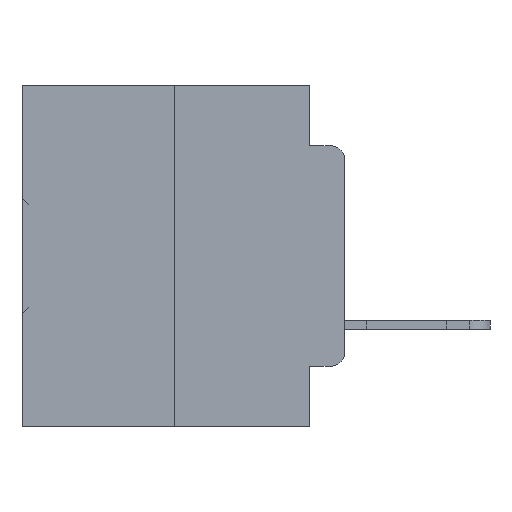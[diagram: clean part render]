
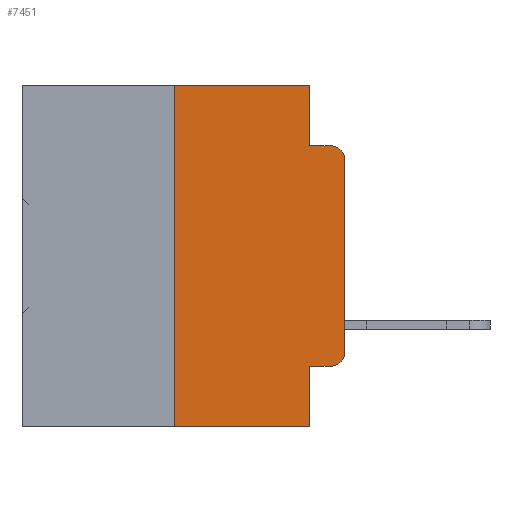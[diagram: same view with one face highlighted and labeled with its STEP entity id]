
A CAD part, left-side view. The second image highlights one B-rep face of the part: STEP entity #7451.
In plain terms, the highlighted planar face has unit normal (-1, 0, 0).
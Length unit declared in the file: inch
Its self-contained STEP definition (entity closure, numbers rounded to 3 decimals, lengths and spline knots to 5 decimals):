
#826 = EDGE_LOOP ( 'NONE', ( #3162, #15771, #3826, #35376, #5031, #7640, #29215, #8530, #10834, #23584 ) ) ;
#985 = VERTEX_POINT ( 'NONE', #22068 ) ;
#1111 = VECTOR ( 'NONE', #28301, 39.37008 ) ;
#1576 = DIRECTION ( 'NONE',  ( 0., 0., -1. ) ) ;
#1656 = DIRECTION ( 'NONE',  ( 0., 0., -1. ) ) ;
#1663 = DIRECTION ( 'NONE',  ( 1., 0., 0. ) ) ;
#1795 = PLANE ( 'NONE',  #16430 ) ;
#1800 = EDGE_CURVE ( 'NONE', #10800, #985, #11108, .T. ) ;
#1982 = VECTOR ( 'NONE', #33667, 39.37008 ) ;
#2269 = CARTESIAN_POINT ( 'NONE',  ( 0., 0.473, 0. ) ) ;
#2577 = VERTEX_POINT ( 'NONE', #4134 ) ;
#2790 = VECTOR ( 'NONE', #16209, 39.37008 ) ;
#3162 = ORIENTED_EDGE ( 'NONE', *, *, #30580, .T. ) ;
#3176 = VECTOR ( 'NONE', #31757, 39.37008 ) ;
#3826 = ORIENTED_EDGE ( 'NONE', *, *, #15657, .F. ) ;
#4134 = CARTESIAN_POINT ( 'NONE',  ( 0., 0.02, -0.4115 ) ) ;
#4499 = LINE ( 'NONE', #11227, #1982 ) ;
#5031 = ORIENTED_EDGE ( 'NONE', *, *, #33778, .F. ) ;
#6151 = DIRECTION ( 'NONE',  ( -1., 0., 0. ) ) ;
#6231 = LINE ( 'NONE', #11171, #27954 ) ;
#6439 = VECTOR ( 'NONE', #30556, 39.37008 ) ;
#6777 = VERTEX_POINT ( 'NONE', #19533 ) ;
#7451 = ADVANCED_FACE ( 'NONE', ( #29694 ), #1795, .F. ) ;
#7640 = ORIENTED_EDGE ( 'NONE', *, *, #33179, .F. ) ;
#8530 = ORIENTED_EDGE ( 'NONE', *, *, #23844, .F. ) ;
#9858 = AXIS2_PLACEMENT_3D ( 'NONE', #35767, #19144, #1576 ) ;
#9992 = DIRECTION ( 'NONE',  ( 0., 0., -1. ) ) ;
#10095 = CARTESIAN_POINT ( 'NONE',  ( 0., 0., 0. ) ) ;
#10226 = CARTESIAN_POINT ( 'NONE',  ( 0., 0.051, 0. ) ) ;
#10239 = CARTESIAN_POINT ( 'NONE',  ( 0., 0.051, -0.0885 ) ) ;
#10748 = LINE ( 'NONE', #10095, #2790 ) ;
#10800 = VERTEX_POINT ( 'NONE', #21002 ) ;
#10834 = ORIENTED_EDGE ( 'NONE', *, *, #22007, .T. ) ;
#11108 = LINE ( 'NONE', #10226, #3176 ) ;
#11171 = CARTESIAN_POINT ( 'NONE',  ( 0., 0.473, -0.5 ) ) ;
#11227 = CARTESIAN_POINT ( 'NONE',  ( 0., 0.473, 0. ) ) ;
#11642 = CARTESIAN_POINT ( 'NONE',  ( 0., 0.25, -0.5 ) ) ;
#12464 = VECTOR ( 'NONE', #18815, 39.37008 ) ;
#14066 = DIRECTION ( 'NONE',  ( 0., -1., 0. ) ) ;
#14170 = CARTESIAN_POINT ( 'NONE',  ( 0., 0.051, -0.4115 ) ) ;
#15144 = LINE ( 'NONE', #10239, #12464 ) ;
#15657 = EDGE_CURVE ( 'NONE', #985, #23692, #15144, .T. ) ;
#15771 = ORIENTED_EDGE ( 'NONE', *, *, #17566, .T. ) ;
#16209 = DIRECTION ( 'NONE',  ( 0., 0., 1. ) ) ;
#16430 = AXIS2_PLACEMENT_3D ( 'NONE', #2269, #1663, #1656 ) ;
#17370 = CARTESIAN_POINT ( 'NONE',  ( 0., 0.25, 0. ) ) ;
#17566 = EDGE_CURVE ( 'NONE', #6777, #23692, #17695, .T. ) ;
#17583 = VERTEX_POINT ( 'NONE', #24711 ) ;
#17695 = CIRCLE ( 'NONE', #9858, 0.02 ) ;
#18350 = CARTESIAN_POINT ( 'NONE',  ( 0., 0.051, 0. ) ) ;
#18743 = AXIS2_PLACEMENT_3D ( 'NONE', #23240, #6151, #26044 ) ;
#18815 = DIRECTION ( 'NONE',  ( 0., -1., 0. ) ) ;
#19144 = DIRECTION ( 'NONE',  ( -1., 0., 0. ) ) ;
#19533 = CARTESIAN_POINT ( 'NONE',  ( 0., 0., -0.1085 ) ) ;
#20837 = EDGE_CURVE ( 'NONE', #2577, #17583, #26599, .T. ) ;
#21002 = CARTESIAN_POINT ( 'NONE',  ( 0., 0.051, 0. ) ) ;
#21502 = VECTOR ( 'NONE', #9992, 39.37008 ) ;
#21652 = LINE ( 'NONE', #27787, #6439 ) ;
#22007 = EDGE_CURVE ( 'NONE', #23308, #2577, #21652, .T. ) ;
#22068 = CARTESIAN_POINT ( 'NONE',  ( 0., 0.051, -0.0885 ) ) ;
#23240 = CARTESIAN_POINT ( 'NONE',  ( 0., 0.02, -0.3915 ) ) ;
#23308 = VERTEX_POINT ( 'NONE', #14170 ) ;
#23584 = ORIENTED_EDGE ( 'NONE', *, *, #20837, .T. ) ;
#23692 = VERTEX_POINT ( 'NONE', #31692 ) ;
#23844 = EDGE_CURVE ( 'NONE', #23308, #30787, #27150, .T. ) ;
#24250 = LINE ( 'NONE', #25527, #1111 ) ;
#24711 = CARTESIAN_POINT ( 'NONE',  ( 0., 0., -0.3915 ) ) ;
#25527 = CARTESIAN_POINT ( 'NONE',  ( 0., 0.25, 0. ) ) ;
#26044 = DIRECTION ( 'NONE',  ( 0., 0., -1. ) ) ;
#26599 = CIRCLE ( 'NONE', #18743, 0.02 ) ;
#27150 = LINE ( 'NONE', #18350, #21502 ) ;
#27787 = CARTESIAN_POINT ( 'NONE',  ( 0., 0.051, -0.4115 ) ) ;
#27954 = VECTOR ( 'NONE', #14066, 39.37008 ) ;
#28125 = CARTESIAN_POINT ( 'NONE',  ( 0., 0.051, -0.5 ) ) ;
#28301 = DIRECTION ( 'NONE',  ( 0., 0., 1. ) ) ;
#29215 = ORIENTED_EDGE ( 'NONE', *, *, #29353, .T. ) ;
#29353 = EDGE_CURVE ( 'NONE', #31983, #30787, #6231, .T. ) ;
#29694 = FACE_OUTER_BOUND ( 'NONE', #826, .T. ) ;
#30142 = VERTEX_POINT ( 'NONE', #17370 ) ;
#30556 = DIRECTION ( 'NONE',  ( 0., -1., 0. ) ) ;
#30580 = EDGE_CURVE ( 'NONE', #17583, #6777, #10748, .T. ) ;
#30787 = VERTEX_POINT ( 'NONE', #28125 ) ;
#31692 = CARTESIAN_POINT ( 'NONE',  ( 0., 0.02, -0.0885 ) ) ;
#31757 = DIRECTION ( 'NONE',  ( 0., 0., -1. ) ) ;
#31983 = VERTEX_POINT ( 'NONE', #11642 ) ;
#33179 = EDGE_CURVE ( 'NONE', #31983, #30142, #24250, .T. ) ;
#33667 = DIRECTION ( 'NONE',  ( 0., -1., 0. ) ) ;
#33778 = EDGE_CURVE ( 'NONE', #30142, #10800, #4499, .T. ) ;
#35376 = ORIENTED_EDGE ( 'NONE', *, *, #1800, .F. ) ;
#35767 = CARTESIAN_POINT ( 'NONE',  ( 0., 0.02, -0.1085 ) ) ;
